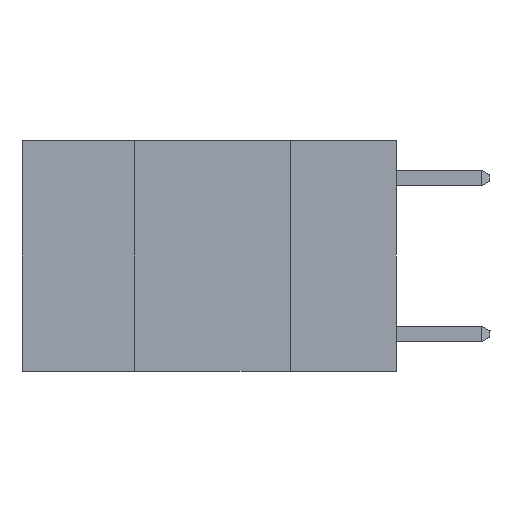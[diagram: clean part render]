
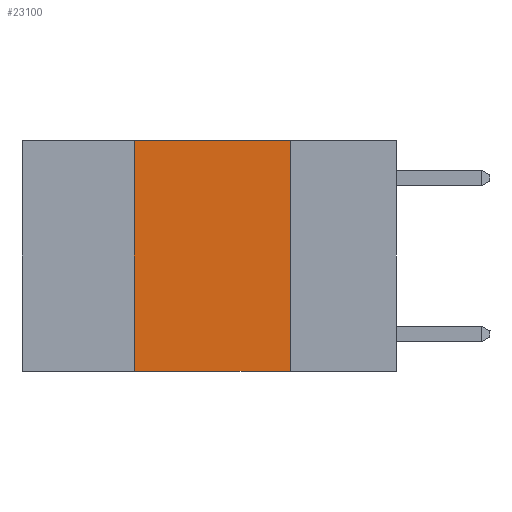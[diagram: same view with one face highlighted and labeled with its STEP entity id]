
A CAD part, left-side view. The second image highlights one B-rep face of the part: STEP entity #23100.
In plain terms, the highlighted planar face has unit normal (-1, 0, 0).
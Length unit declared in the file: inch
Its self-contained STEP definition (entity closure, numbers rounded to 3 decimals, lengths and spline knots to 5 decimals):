
#846 = ORIENTED_EDGE ( 'NONE', *, *, #20925, .F. ) ;
#1824 = DIRECTION ( 'NONE',  ( 0., 0., 1. ) ) ;
#1871 = ORIENTED_EDGE ( 'NONE', *, *, #10951, .T. ) ;
#4823 = LINE ( 'NONE', #14887, #29182 ) ;
#5965 = LINE ( 'NONE', #8181, #29483 ) ;
#6754 = ORIENTED_EDGE ( 'NONE', *, *, #20528, .F. ) ;
#7498 = CARTESIAN_POINT ( 'NONE',  ( 0., 0.42, -0.37 ) ) ;
#7861 = EDGE_LOOP ( 'NONE', ( #6754, #29776, #846, #1871 ) ) ;
#8181 = CARTESIAN_POINT ( 'NONE',  ( 0., 0.6, 0. ) ) ;
#9164 = CARTESIAN_POINT ( 'NONE',  ( 0., 0.42, 0. ) ) ;
#9495 = CARTESIAN_POINT ( 'NONE',  ( 0., 0.6, 0. ) ) ;
#9570 = CARTESIAN_POINT ( 'NONE',  ( 0., 0.17, -0.37 ) ) ;
#9633 = VERTEX_POINT ( 'NONE', #17894 ) ;
#10620 = DIRECTION ( 'NONE',  ( 0., -1., 0. ) ) ;
#10951 = EDGE_CURVE ( 'NONE', #11914, #19664, #23741, .T. ) ;
#11914 = VERTEX_POINT ( 'NONE', #7498 ) ;
#13788 = CARTESIAN_POINT ( 'NONE',  ( 0., 0.6, -0.37 ) ) ;
#14239 = PLANE ( 'NONE',  #16624 ) ;
#14339 = DIRECTION ( 'NONE',  ( 1., 0., 0. ) ) ;
#14887 = CARTESIAN_POINT ( 'NONE',  ( 0., 0.17, 0. ) ) ;
#14988 = DIRECTION ( 'NONE',  ( 0., 0., -1. ) ) ;
#15341 = FACE_OUTER_BOUND ( 'NONE', #7861, .T. ) ;
#16624 = AXIS2_PLACEMENT_3D ( 'NONE', #9495, #14339, #30459 ) ;
#16906 = EDGE_CURVE ( 'NONE', #21242, #9633, #5965, .T. ) ;
#17549 = CARTESIAN_POINT ( 'NONE',  ( 0., 0.42, 0. ) ) ;
#17894 = CARTESIAN_POINT ( 'NONE',  ( 0., 0.17, 0. ) ) ;
#18384 = VECTOR ( 'NONE', #1824, 39.37008 ) ;
#19664 = VERTEX_POINT ( 'NONE', #9570 ) ;
#20528 = EDGE_CURVE ( 'NONE', #9633, #19664, #4823, .T. ) ;
#20925 = EDGE_CURVE ( 'NONE', #11914, #21242, #24562, .T. ) ;
#21242 = VERTEX_POINT ( 'NONE', #17549 ) ;
#23100 = ADVANCED_FACE ( 'NONE', ( #15341 ), #14239, .F. ) ;
#23741 = LINE ( 'NONE', #13788, #29064 ) ;
#24562 = LINE ( 'NONE', #9164, #18384 ) ;
#29064 = VECTOR ( 'NONE', #30055, 39.37008 ) ;
#29182 = VECTOR ( 'NONE', #14988, 39.37008 ) ;
#29483 = VECTOR ( 'NONE', #10620, 39.37008 ) ;
#29776 = ORIENTED_EDGE ( 'NONE', *, *, #16906, .F. ) ;
#30055 = DIRECTION ( 'NONE',  ( 0., -1., 0. ) ) ;
#30459 = DIRECTION ( 'NONE',  ( 0., 0., -1. ) ) ;
